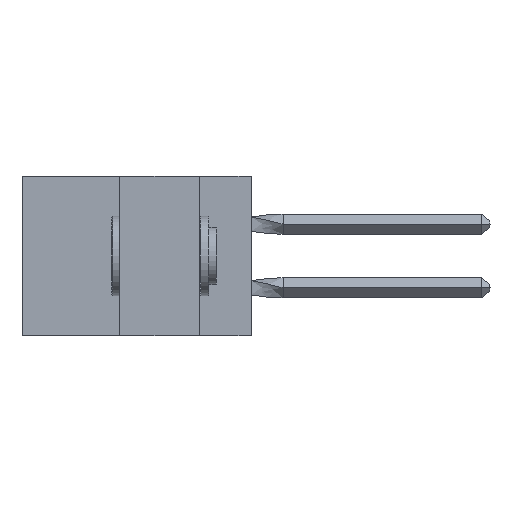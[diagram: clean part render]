
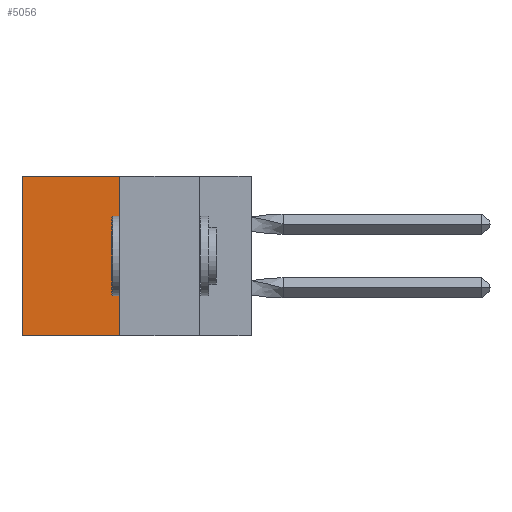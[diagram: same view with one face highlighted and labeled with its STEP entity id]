
A CAD part, left-side view. The second image highlights one B-rep face of the part: STEP entity #5056.
In plain terms, the highlighted planar face has unit normal (-1, 0, 0).
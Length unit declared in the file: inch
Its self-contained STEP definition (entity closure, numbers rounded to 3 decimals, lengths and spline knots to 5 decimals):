
#596 = CARTESIAN_POINT ( 'NONE',  ( 0.305, 0.72, -0.5 ) ) ;
#1550 = ORIENTED_EDGE ( 'NONE', *, *, #11180, .F. ) ;
#2090 = CARTESIAN_POINT ( 'NONE',  ( 0.305, 0.72, -0.5 ) ) ;
#2754 = VECTOR ( 'NONE', #13390, 39.37008 ) ;
#3135 = EDGE_CURVE ( 'NONE', #14881, #16933, #6479, .T. ) ;
#3308 = DIRECTION ( 'NONE',  ( 1., 0., 0. ) ) ;
#3780 = ORIENTED_EDGE ( 'NONE', *, *, #5148, .F. ) ;
#4211 = VERTEX_POINT ( 'NONE', #12051 ) ;
#4302 = DIRECTION ( 'NONE',  ( 0., 0., -1. ) ) ;
#4804 = VECTOR ( 'NONE', #9634, 39.37008 ) ;
#5056 = ADVANCED_FACE ( 'NONE', ( #18064 ), #11884, .F. ) ;
#5148 = EDGE_CURVE ( 'NONE', #14953, #4211, #10124, .T. ) ;
#5525 = VECTOR ( 'NONE', #4302, 39.37008 ) ;
#6265 = DIRECTION ( 'NONE',  ( 0., 0., -1. ) ) ;
#6479 = LINE ( 'NONE', #596, #2754 ) ;
#7199 = DIRECTION ( 'NONE',  ( 0., 1., 0. ) ) ;
#7266 = EDGE_CURVE ( 'NONE', #14953, #14881, #17762, .T. ) ;
#7420 = ORIENTED_EDGE ( 'NONE', *, *, #7266, .T. ) ;
#8072 = CARTESIAN_POINT ( 'NONE',  ( 0.305, 0.413, -0.5 ) ) ;
#8971 = CARTESIAN_POINT ( 'NONE',  ( 0.305, 0.413, -0.5 ) ) ;
#9634 = DIRECTION ( 'NONE',  ( 0., 1., 0. ) ) ;
#9877 = CARTESIAN_POINT ( 'NONE',  ( 0.305, 0.413, 0. ) ) ;
#10124 = LINE ( 'NONE', #16785, #5525 ) ;
#10267 = VECTOR ( 'NONE', #7199, 39.37008 ) ;
#11180 = EDGE_CURVE ( 'NONE', #4211, #16933, #15562, .T. ) ;
#11884 = PLANE ( 'NONE',  #14800 ) ;
#12051 = CARTESIAN_POINT ( 'NONE',  ( 0.305, 0.413, -0.5 ) ) ;
#13390 = DIRECTION ( 'NONE',  ( 0., 0., -1. ) ) ;
#14800 = AXIS2_PLACEMENT_3D ( 'NONE', #8971, #3308, #6265 ) ;
#14881 = VERTEX_POINT ( 'NONE', #17868 ) ;
#14953 = VERTEX_POINT ( 'NONE', #18085 ) ;
#15029 = EDGE_LOOP ( 'NONE', ( #16183, #1550, #3780, #7420 ) ) ;
#15562 = LINE ( 'NONE', #8072, #4804 ) ;
#16183 = ORIENTED_EDGE ( 'NONE', *, *, #3135, .T. ) ;
#16785 = CARTESIAN_POINT ( 'NONE',  ( 0.305, 0.413, -0.5 ) ) ;
#16933 = VERTEX_POINT ( 'NONE', #2090 ) ;
#17762 = LINE ( 'NONE', #9877, #10267 ) ;
#17868 = CARTESIAN_POINT ( 'NONE',  ( 0.305, 0.72, 0. ) ) ;
#18064 = FACE_OUTER_BOUND ( 'NONE', #15029, .T. ) ;
#18085 = CARTESIAN_POINT ( 'NONE',  ( 0.305, 0.413, 0. ) ) ;
